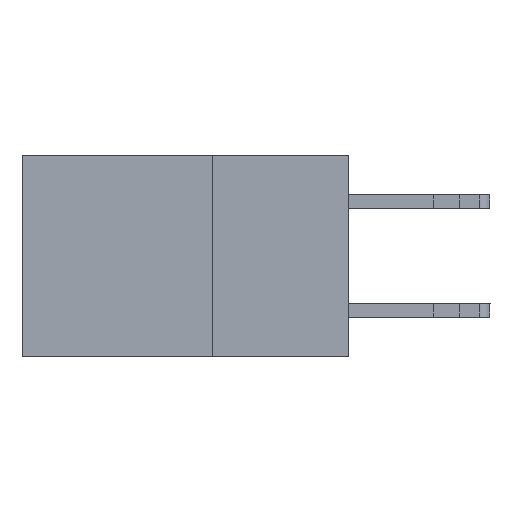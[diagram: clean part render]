
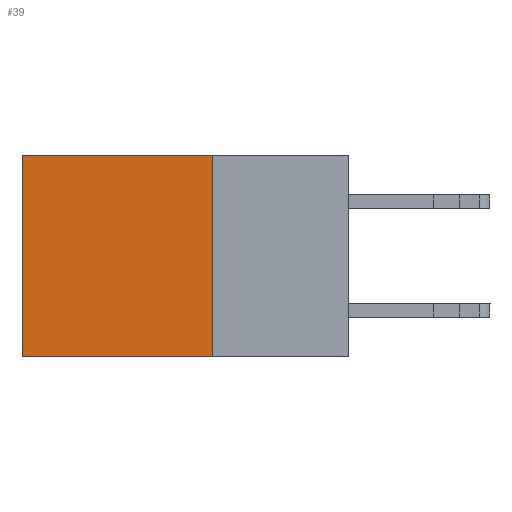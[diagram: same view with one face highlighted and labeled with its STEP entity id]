
A CAD part, left-side view. The second image highlights one B-rep face of the part: STEP entity #39.
In plain terms, the highlighted planar face has unit normal (-1, 0, 0).
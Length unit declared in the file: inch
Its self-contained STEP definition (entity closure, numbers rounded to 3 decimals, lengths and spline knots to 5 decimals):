
#39 = ADVANCED_FACE ( 'NONE', ( #9848 ), #769, .F. ) ;
#769 = PLANE ( 'NONE',  #17175 ) ;
#952 = VERTEX_POINT ( 'NONE', #1567 ) ;
#1567 = CARTESIAN_POINT ( 'NONE',  ( 0.298, 0.6, -0.37 ) ) ;
#1844 = CARTESIAN_POINT ( 'NONE',  ( 0.298, 0.25, 0. ) ) ;
#3094 = EDGE_CURVE ( 'NONE', #13617, #952, #16445, .T. ) ;
#3682 = VECTOR ( 'NONE', #5530, 39.37008 ) ;
#3815 = CARTESIAN_POINT ( 'NONE',  ( 0.298, 0.6, 0. ) ) ;
#3949 = DIRECTION ( 'NONE',  ( 0., 0., -1. ) ) ;
#3976 = VERTEX_POINT ( 'NONE', #14739 ) ;
#4363 = LINE ( 'NONE', #1844, #13149 ) ;
#4727 = CARTESIAN_POINT ( 'NONE',  ( 0.298, 0.25, -0.37 ) ) ;
#5530 = DIRECTION ( 'NONE',  ( 0., 0., -1. ) ) ;
#5782 = DIRECTION ( 'NONE',  ( 0., 1., 0. ) ) ;
#6950 = ORIENTED_EDGE ( 'NONE', *, *, #16633, .F. ) ;
#7120 = LINE ( 'NONE', #13591, #15249 ) ;
#9008 = DIRECTION ( 'NONE',  ( 0., 1., 0. ) ) ;
#9205 = ORIENTED_EDGE ( 'NONE', *, *, #12622, .T. ) ;
#9825 = EDGE_LOOP ( 'NONE', ( #13744, #6950, #11728, #9205 ) ) ;
#9848 = FACE_OUTER_BOUND ( 'NONE', #9825, .T. ) ;
#10980 = DIRECTION ( 'NONE',  ( 1., 0., 0. ) ) ;
#11035 = VECTOR ( 'NONE', #5782, 39.37008 ) ;
#11728 = ORIENTED_EDGE ( 'NONE', *, *, #15489, .F. ) ;
#12513 = CARTESIAN_POINT ( 'NONE',  ( 0.298, 0.6, 0. ) ) ;
#12622 = EDGE_CURVE ( 'NONE', #3976, #13617, #4363, .T. ) ;
#13149 = VECTOR ( 'NONE', #9008, 39.37008 ) ;
#13413 = DIRECTION ( 'NONE',  ( 0., 0., -1. ) ) ;
#13591 = CARTESIAN_POINT ( 'NONE',  ( 0.298, 0.25, 0. ) ) ;
#13617 = VERTEX_POINT ( 'NONE', #3815 ) ;
#13744 = ORIENTED_EDGE ( 'NONE', *, *, #3094, .T. ) ;
#13932 = VERTEX_POINT ( 'NONE', #4727 ) ;
#14739 = CARTESIAN_POINT ( 'NONE',  ( 0.298, 0.25, 0. ) ) ;
#14749 = LINE ( 'NONE', #17023, #11035 ) ;
#15249 = VECTOR ( 'NONE', #13413, 39.37008 ) ;
#15489 = EDGE_CURVE ( 'NONE', #3976, #13932, #7120, .T. ) ;
#16182 = CARTESIAN_POINT ( 'NONE',  ( 0.298, 0.25, 0. ) ) ;
#16445 = LINE ( 'NONE', #12513, #3682 ) ;
#16633 = EDGE_CURVE ( 'NONE', #13932, #952, #14749, .T. ) ;
#17023 = CARTESIAN_POINT ( 'NONE',  ( 0.298, 0.25, -0.37 ) ) ;
#17175 = AXIS2_PLACEMENT_3D ( 'NONE', #16182, #10980, #3949 ) ;
